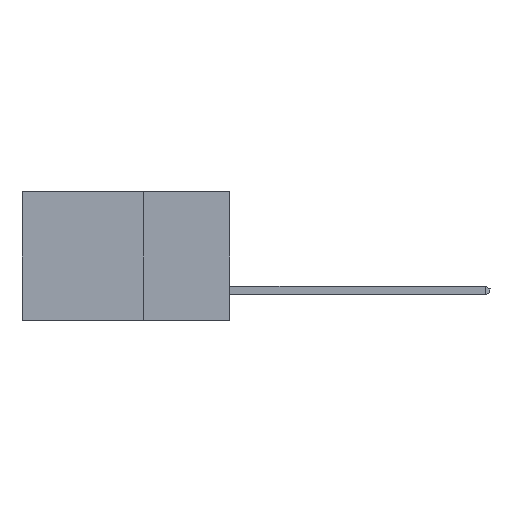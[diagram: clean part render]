
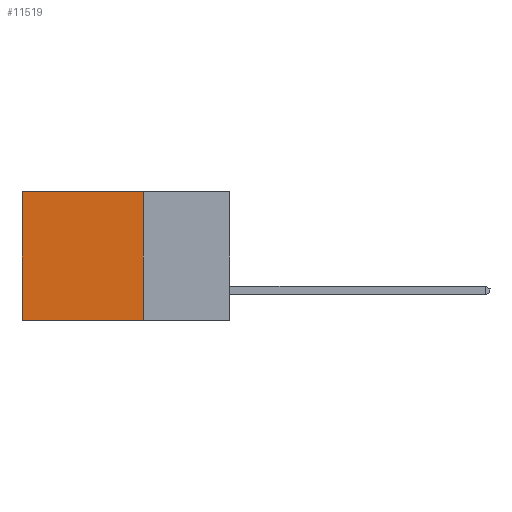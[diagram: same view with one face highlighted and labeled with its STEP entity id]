
A CAD part, left-side view. The second image highlights one B-rep face of the part: STEP entity #11519.
In plain terms, the highlighted planar face has unit normal (-1, 0, 0).
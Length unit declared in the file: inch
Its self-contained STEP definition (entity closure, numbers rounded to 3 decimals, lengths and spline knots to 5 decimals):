
#396 = LINE ( 'NONE', #8152, #18917 ) ;
#1267 = LINE ( 'NONE', #10182, #14076 ) ;
#2491 = VERTEX_POINT ( 'NONE', #4300 ) ;
#3110 = DIRECTION ( 'NONE',  ( 0., 0., -1. ) ) ;
#3976 = EDGE_CURVE ( 'NONE', #10286, #15124, #396, .T. ) ;
#4096 = VERTEX_POINT ( 'NONE', #22647 ) ;
#4300 = CARTESIAN_POINT ( 'NONE',  ( 0.2615, 0.25, 0. ) ) ;
#4880 = CARTESIAN_POINT ( 'NONE',  ( 0.2615, 0.25, -0.37 ) ) ;
#7455 = ORIENTED_EDGE ( 'NONE', *, *, #22114, .T. ) ;
#7759 = CARTESIAN_POINT ( 'NONE',  ( 0.2615, 0.25, -0.37 ) ) ;
#8152 = CARTESIAN_POINT ( 'NONE',  ( 0.2615, 0.25, -0.37 ) ) ;
#8813 = DIRECTION ( 'NONE',  ( 0., 1., 0. ) ) ;
#8928 = CARTESIAN_POINT ( 'NONE',  ( 0.2615, 0.6, -0.37 ) ) ;
#9551 = DIRECTION ( 'NONE',  ( 1., 0., 0. ) ) ;
#9807 = EDGE_CURVE ( 'NONE', #2491, #4096, #1267, .T. ) ;
#10182 = CARTESIAN_POINT ( 'NONE',  ( 0.2615, 0.25, 0. ) ) ;
#10251 = LINE ( 'NONE', #8928, #19020 ) ;
#10286 = VERTEX_POINT ( 'NONE', #7759 ) ;
#10457 = ORIENTED_EDGE ( 'NONE', *, *, #9807, .T. ) ;
#10641 = FACE_OUTER_BOUND ( 'NONE', #18816, .T. ) ;
#11519 = ADVANCED_FACE ( 'NONE', ( #10641 ), #13143, .F. ) ;
#11833 = ORIENTED_EDGE ( 'NONE', *, *, #3976, .F. ) ;
#13143 = PLANE ( 'NONE',  #19196 ) ;
#14076 = VECTOR ( 'NONE', #22481, 39.37008 ) ;
#15124 = VERTEX_POINT ( 'NONE', #15591 ) ;
#15591 = CARTESIAN_POINT ( 'NONE',  ( 0.2615, 0.6, -0.37 ) ) ;
#17705 = EDGE_CURVE ( 'NONE', #2491, #10286, #22869, .T. ) ;
#18352 = ORIENTED_EDGE ( 'NONE', *, *, #17705, .F. ) ;
#18816 = EDGE_LOOP ( 'NONE', ( #7455, #11833, #18352, #10457 ) ) ;
#18917 = VECTOR ( 'NONE', #8813, 39.37008 ) ;
#19020 = VECTOR ( 'NONE', #22935, 39.37008 ) ;
#19196 = AXIS2_PLACEMENT_3D ( 'NONE', #20072, #9551, #21804 ) ;
#20072 = CARTESIAN_POINT ( 'NONE',  ( 0.2615, 0.25, -0.37 ) ) ;
#21804 = DIRECTION ( 'NONE',  ( 0., 0., -1. ) ) ;
#22114 = EDGE_CURVE ( 'NONE', #4096, #15124, #10251, .T. ) ;
#22336 = VECTOR ( 'NONE', #3110, 39.37008 ) ;
#22481 = DIRECTION ( 'NONE',  ( 0., 1., 0. ) ) ;
#22647 = CARTESIAN_POINT ( 'NONE',  ( 0.2615, 0.6, 0. ) ) ;
#22869 = LINE ( 'NONE', #4880, #22336 ) ;
#22935 = DIRECTION ( 'NONE',  ( 0., 0., -1. ) ) ;
